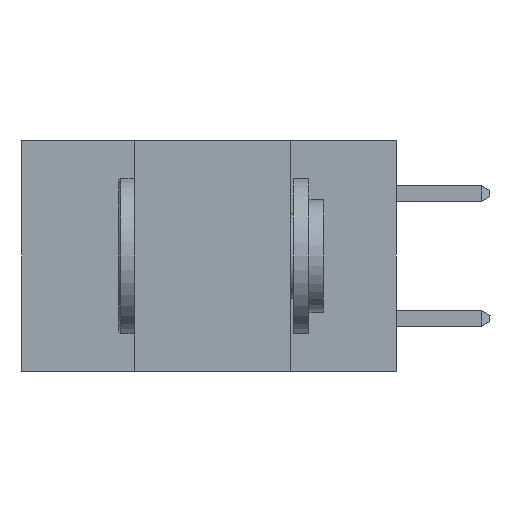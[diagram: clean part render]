
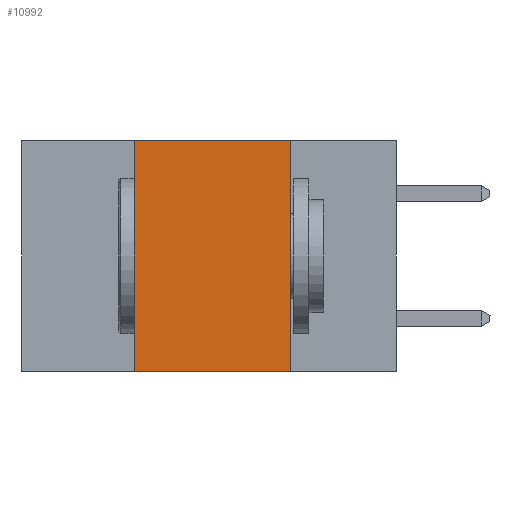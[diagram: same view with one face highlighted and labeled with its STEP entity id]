
A CAD part, left-side view. The second image highlights one B-rep face of the part: STEP entity #10992.
In plain terms, the highlighted planar face has unit normal (-1, 0, 0).
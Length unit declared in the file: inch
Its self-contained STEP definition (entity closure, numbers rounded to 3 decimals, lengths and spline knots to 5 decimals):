
#405 = FACE_OUTER_BOUND ( 'NONE', #9162, .T. ) ;
#559 = EDGE_CURVE ( 'NONE', #10328, #12791, #11801, .T. ) ;
#1611 = ORIENTED_EDGE ( 'NONE', *, *, #7582, .F. ) ;
#2528 = EDGE_CURVE ( 'NONE', #10328, #5536, #12809, .T. ) ;
#2642 = CARTESIAN_POINT ( 'NONE',  ( 0., 0.17, -0.37 ) ) ;
#3311 = ORIENTED_EDGE ( 'NONE', *, *, #559, .F. ) ;
#4665 = ORIENTED_EDGE ( 'NONE', *, *, #12279, .F. ) ;
#5407 = DIRECTION ( 'NONE',  ( 0., 0., 1. ) ) ;
#5536 = VERTEX_POINT ( 'NONE', #2642 ) ;
#5715 = ORIENTED_EDGE ( 'NONE', *, *, #2528, .T. ) ;
#6212 = CARTESIAN_POINT ( 'NONE',  ( 0., 0.42, -0.37 ) ) ;
#7582 = EDGE_CURVE ( 'NONE', #12144, #5536, #14838, .T. ) ;
#8062 = VECTOR ( 'NONE', #5407, 39.37008 ) ;
#8646 = CARTESIAN_POINT ( 'NONE',  ( 0., 0.42, -0.37 ) ) ;
#8987 = DIRECTION ( 'NONE',  ( 0., 0., -1. ) ) ;
#9008 = CARTESIAN_POINT ( 'NONE',  ( 0., 0.42, 0. ) ) ;
#9012 = CARTESIAN_POINT ( 'NONE',  ( 0., 0.6, 0. ) ) ;
#9162 = EDGE_LOOP ( 'NONE', ( #1611, #4665, #3311, #5715 ) ) ;
#9913 = LINE ( 'NONE', #9012, #16781 ) ;
#10328 = VERTEX_POINT ( 'NONE', #8646 ) ;
#10992 = ADVANCED_FACE ( 'NONE', ( #405 ), #15900, .F. ) ;
#11142 = VECTOR ( 'NONE', #13464, 39.37008 ) ;
#11417 = DIRECTION ( 'NONE',  ( 0., -1., 0. ) ) ;
#11547 = CARTESIAN_POINT ( 'NONE',  ( 0., 0.6, -0.37 ) ) ;
#11777 = CARTESIAN_POINT ( 'NONE',  ( 0., 0.6, 0. ) ) ;
#11801 = LINE ( 'NONE', #6212, #8062 ) ;
#12144 = VERTEX_POINT ( 'NONE', #14263 ) ;
#12279 = EDGE_CURVE ( 'NONE', #12791, #12144, #9913, .T. ) ;
#12387 = VECTOR ( 'NONE', #11417, 39.37008 ) ;
#12791 = VERTEX_POINT ( 'NONE', #9008 ) ;
#12809 = LINE ( 'NONE', #11547, #12387 ) ;
#13464 = DIRECTION ( 'NONE',  ( 0., 0., -1. ) ) ;
#13481 = CARTESIAN_POINT ( 'NONE',  ( 0., 0.17, -0.37 ) ) ;
#14263 = CARTESIAN_POINT ( 'NONE',  ( 0., 0.17, 0. ) ) ;
#14838 = LINE ( 'NONE', #13481, #11142 ) ;
#15900 = PLANE ( 'NONE',  #16355 ) ;
#15921 = DIRECTION ( 'NONE',  ( 0., -1., 0. ) ) ;
#16355 = AXIS2_PLACEMENT_3D ( 'NONE', #11777, #17231, #8987 ) ;
#16781 = VECTOR ( 'NONE', #15921, 39.37008 ) ;
#17231 = DIRECTION ( 'NONE',  ( 1., 0., 0. ) ) ;
